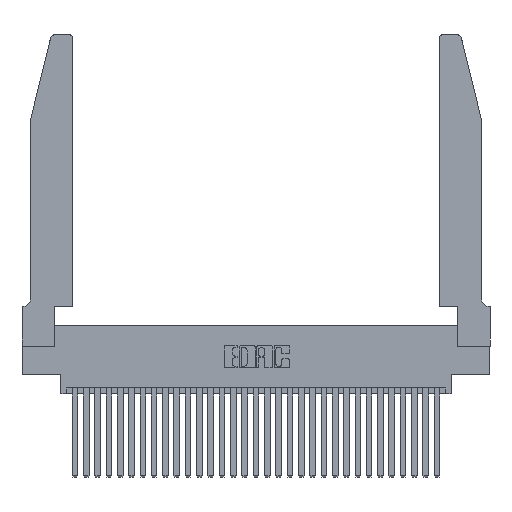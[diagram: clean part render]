
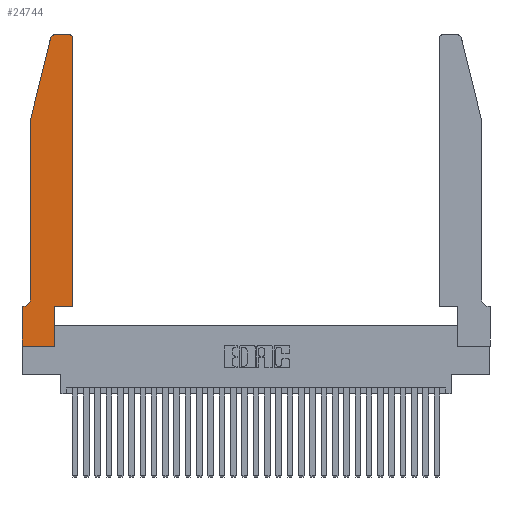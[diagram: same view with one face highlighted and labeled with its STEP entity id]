
A CAD part, top view. The second image highlights one B-rep face of the part: STEP entity #24744.
In plain terms, the highlighted planar face has unit normal (0, 0, 1).
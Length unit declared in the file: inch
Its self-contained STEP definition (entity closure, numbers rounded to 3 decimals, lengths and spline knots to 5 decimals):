
#422 = CARTESIAN_POINT ( 'NONE',  ( 0.0755, 2., 0.37 ) ) ;
#580 = CARTESIAN_POINT ( 'NONE',  ( 0.4505, 0.35, 0.37 ) ) ;
#917 = VERTEX_POINT ( 'NONE', #17722 ) ;
#1071 = CARTESIAN_POINT ( 'NONE',  ( 0., 0., 0.37 ) ) ;
#1360 = VERTEX_POINT ( 'NONE', #19296 ) ;
#1380 = EDGE_CURVE ( 'NONE', #917, #16960, #24201, .T. ) ;
#1533 = DIRECTION ( 'NONE',  ( -0.239, -0.971, 0. ) ) ;
#2472 = VERTEX_POINT ( 'NONE', #16572 ) ;
#2649 = LINE ( 'NONE', #11619, #23015 ) ;
#3532 = EDGE_CURVE ( 'NONE', #13028, #2472, #28719, .T. ) ;
#3558 = DIRECTION ( 'NONE',  ( 0., -1., 0. ) ) ;
#3768 = FACE_OUTER_BOUND ( 'NONE', #10226, .T. ) ;
#4142 = CARTESIAN_POINT ( 'NONE',  ( 0.0755, 0.42, 0.37 ) ) ;
#4342 = ORIENTED_EDGE ( 'NONE', *, *, #24804, .T. ) ;
#4432 = VERTEX_POINT ( 'NONE', #26090 ) ;
#4785 = VERTEX_POINT ( 'NONE', #10699 ) ;
#6096 = VECTOR ( 'NONE', #10116, 39.37008 ) ;
#6125 = CIRCLE ( 'NONE', #7495, 0.07 ) ;
#6174 = DIRECTION ( 'NONE',  ( 0., 0., -1. ) ) ;
#6903 = LINE ( 'NONE', #580, #13043 ) ;
#7098 = CARTESIAN_POINT ( 'NONE',  ( 0.0755, 0.35, 0.37 ) ) ;
#7185 = CARTESIAN_POINT ( 'NONE',  ( 0.2865, 0., 0.37 ) ) ;
#7495 = AXIS2_PLACEMENT_3D ( 'NONE', #18562, #6174, #23527 ) ;
#7641 = ORIENTED_EDGE ( 'NONE', *, *, #18605, .T. ) ;
#7749 = DIRECTION ( 'NONE',  ( 1., 0., 0. ) ) ;
#7772 = CARTESIAN_POINT ( 'NONE',  ( 0.2605, 2.75, 0.37 ) ) ;
#7797 = EDGE_CURVE ( 'NONE', #2472, #19611, #23421, .T. ) ;
#7815 = DIRECTION ( 'NONE',  ( 0., 0., 1. ) ) ;
#8984 = VERTEX_POINT ( 'NONE', #26859 ) ;
#9232 = LINE ( 'NONE', #9921, #24575 ) ;
#9396 = CIRCLE ( 'NONE', #13790, 0.03 ) ;
#9921 = CARTESIAN_POINT ( 'NONE',  ( 0., 0., 0.37 ) ) ;
#10116 = DIRECTION ( 'NONE',  ( 0., 1., 0. ) ) ;
#10119 = PLANE ( 'NONE',  #15720 ) ;
#10226 = EDGE_LOOP ( 'NONE', ( #23201, #24583, #18943, #21338, #25578, #25727, #4342, #25799, #24071, #7641, #13520, #26451 ) ) ;
#10420 = DIRECTION ( 'NONE',  ( 0., 0., 1. ) ) ;
#10680 = VERTEX_POINT ( 'NONE', #16348 ) ;
#10699 = CARTESIAN_POINT ( 'NONE',  ( 0.25487, 2.72718, 0.37 ) ) ;
#11619 = CARTESIAN_POINT ( 'NONE',  ( 0.0755, 2., 0.37 ) ) ;
#11665 = EDGE_CURVE ( 'NONE', #19611, #4785, #9396, .T. ) ;
#12647 = DIRECTION ( 'NONE',  ( 1., 0., 0. ) ) ;
#12749 = CARTESIAN_POINT ( 'NONE',  ( 0.284, 2.72, 0.37 ) ) ;
#13028 = VERTEX_POINT ( 'NONE', #18690 ) ;
#13043 = VECTOR ( 'NONE', #22802, 39.37008 ) ;
#13451 = VECTOR ( 'NONE', #31379, 39.37008 ) ;
#13520 = ORIENTED_EDGE ( 'NONE', *, *, #29344, .T. ) ;
#13790 = AXIS2_PLACEMENT_3D ( 'NONE', #12749, #7815, #22411 ) ;
#15146 = CARTESIAN_POINT ( 'NONE',  ( 0., 0.35, 0.37 ) ) ;
#15449 = CARTESIAN_POINT ( 'NONE',  ( 0.4205, 2.72, 0.37 ) ) ;
#15612 = CARTESIAN_POINT ( 'NONE',  ( 0.284, 2.75, 0.37 ) ) ;
#15720 = AXIS2_PLACEMENT_3D ( 'NONE', #15146, #19838, #7749 ) ;
#16090 = CARTESIAN_POINT ( 'NONE',  ( 0.4505, 0.35, 0.37 ) ) ;
#16301 = EDGE_CURVE ( 'NONE', #1360, #31026, #9232, .T. ) ;
#16348 = CARTESIAN_POINT ( 'NONE',  ( 0.4505, 0.35, 0.37 ) ) ;
#16572 = CARTESIAN_POINT ( 'NONE',  ( 0.4205, 2.75, 0.37 ) ) ;
#16960 = VERTEX_POINT ( 'NONE', #30065 ) ;
#17383 = CARTESIAN_POINT ( 'NONE',  ( 0.2865, 0.35, 0.37 ) ) ;
#17722 = CARTESIAN_POINT ( 'NONE',  ( 0.0055, 0.35, 0.37 ) ) ;
#17985 = VERTEX_POINT ( 'NONE', #4142 ) ;
#18419 = VECTOR ( 'NONE', #19712, 39.37008 ) ;
#18539 = DIRECTION ( 'NONE',  ( 1., 0., 0. ) ) ;
#18562 = CARTESIAN_POINT ( 'NONE',  ( 0.0055, 0.42, 0.37 ) ) ;
#18605 = EDGE_CURVE ( 'NONE', #4432, #10680, #26105, .T. ) ;
#18690 = CARTESIAN_POINT ( 'NONE',  ( 0.4505, 2.72, 0.37 ) ) ;
#18943 = ORIENTED_EDGE ( 'NONE', *, *, #29571, .T. ) ;
#19296 = CARTESIAN_POINT ( 'NONE',  ( 0., 0., 0.37 ) ) ;
#19458 = LINE ( 'NONE', #1071, #27169 ) ;
#19611 = VERTEX_POINT ( 'NONE', #15612 ) ;
#19712 = DIRECTION ( 'NONE',  ( 0., -1., 0. ) ) ;
#19838 = DIRECTION ( 'NONE',  ( 0., 0., 1. ) ) ;
#21338 = ORIENTED_EDGE ( 'NONE', *, *, #23351, .T. ) ;
#21872 = LINE ( 'NONE', #422, #18419 ) ;
#22411 = DIRECTION ( 'NONE',  ( 1., 0., 0. ) ) ;
#22698 = DIRECTION ( 'NONE',  ( -1., 0., 0. ) ) ;
#22802 = DIRECTION ( 'NONE',  ( 0., 1., 0. ) ) ;
#23015 = VECTOR ( 'NONE', #1533, 39.37008 ) ;
#23201 = ORIENTED_EDGE ( 'NONE', *, *, #7797, .T. ) ;
#23351 = EDGE_CURVE ( 'NONE', #8984, #17985, #21872, .T. ) ;
#23421 = LINE ( 'NONE', #7772, #25313 ) ;
#23527 = DIRECTION ( 'NONE',  ( -1., 0., 0. ) ) ;
#24071 = ORIENTED_EDGE ( 'NONE', *, *, #30449, .T. ) ;
#24175 = EDGE_CURVE ( 'NONE', #17985, #917, #6125, .T. ) ;
#24201 = LINE ( 'NONE', #7098, #13451 ) ;
#24248 = VECTOR ( 'NONE', #18539, 39.37008 ) ;
#24575 = VECTOR ( 'NONE', #24829, 39.37008 ) ;
#24583 = ORIENTED_EDGE ( 'NONE', *, *, #11665, .T. ) ;
#24744 = ADVANCED_FACE ( 'NONE', ( #3768 ), #10119, .T. ) ;
#24804 = EDGE_CURVE ( 'NONE', #16960, #1360, #19458, .T. ) ;
#24829 = DIRECTION ( 'NONE',  ( 1., 0., 0. ) ) ;
#25313 = VECTOR ( 'NONE', #22698, 39.37008 ) ;
#25578 = ORIENTED_EDGE ( 'NONE', *, *, #24175, .T. ) ;
#25727 = ORIENTED_EDGE ( 'NONE', *, *, #1380, .T. ) ;
#25799 = ORIENTED_EDGE ( 'NONE', *, *, #16301, .T. ) ;
#26090 = CARTESIAN_POINT ( 'NONE',  ( 0.2865, 0.35, 0.37 ) ) ;
#26105 = LINE ( 'NONE', #16090, #24248 ) ;
#26451 = ORIENTED_EDGE ( 'NONE', *, *, #3532, .T. ) ;
#26859 = CARTESIAN_POINT ( 'NONE',  ( 0.0755, 2., 0.37 ) ) ;
#27169 = VECTOR ( 'NONE', #3558, 39.37008 ) ;
#27969 = LINE ( 'NONE', #17383, #6096 ) ;
#28719 = CIRCLE ( 'NONE', #28894, 0.03 ) ;
#28894 = AXIS2_PLACEMENT_3D ( 'NONE', #15449, #10420, #12647 ) ;
#29344 = EDGE_CURVE ( 'NONE', #10680, #13028, #6903, .T. ) ;
#29571 = EDGE_CURVE ( 'NONE', #4785, #8984, #2649, .T. ) ;
#30065 = CARTESIAN_POINT ( 'NONE',  ( 0., 0.35, 0.37 ) ) ;
#30449 = EDGE_CURVE ( 'NONE', #31026, #4432, #27969, .T. ) ;
#31026 = VERTEX_POINT ( 'NONE', #7185 ) ;
#31379 = DIRECTION ( 'NONE',  ( -1., 0., 0. ) ) ;
